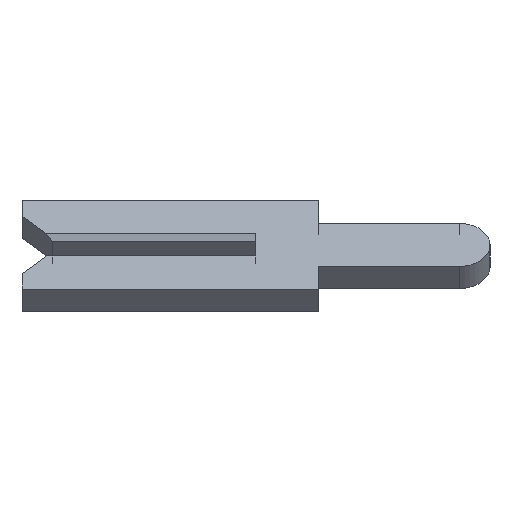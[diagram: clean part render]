
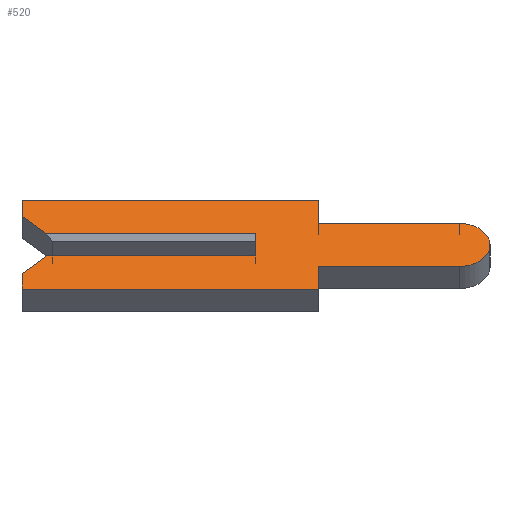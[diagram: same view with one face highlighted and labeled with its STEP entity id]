
A CAD part, left-side view. The second image highlights one B-rep face of the part: STEP entity #520.
In plain terms, the highlighted face is planar.
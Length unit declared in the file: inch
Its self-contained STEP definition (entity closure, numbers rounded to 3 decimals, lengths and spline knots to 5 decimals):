
#5 = VERTEX_POINT ( 'NONE', #179 ) ;
#6 = EDGE_CURVE ( 'NONE', #775, #765, #870, .T. ) ;
#57 = LINE ( 'NONE', #976, #354 ) ;
#66 = DIRECTION ( 'NONE',  ( 0., 0., 1. ) ) ;
#78 = ORIENTED_EDGE ( 'NONE', *, *, #1121, .F. ) ;
#79 = VECTOR ( 'NONE', #904, 39.37008 ) ;
#104 = LINE ( 'NONE', #142, #143 ) ;
#142 = CARTESIAN_POINT ( 'NONE',  ( -0.01, -0.1305, -0.01 ) ) ;
#143 = VECTOR ( 'NONE', #696, 39.37008 ) ;
#173 = VERTEX_POINT ( 'NONE', #862 ) ;
#179 = CARTESIAN_POINT ( 'NONE',  ( -0.01, -0.04, 0.0195 ) ) ;
#180 = EDGE_CURVE ( 'NONE', #813, #1095, #745, .T. ) ;
#182 = CARTESIAN_POINT ( 'NONE',  ( -0.01, 0.15, 0.026 ) ) ;
#183 = CARTESIAN_POINT ( 'NONE',  ( -0.01, 0., -0.01 ) ) ;
#207 = PLANE ( 'NONE',  #774 ) ;
#228 = ORIENTED_EDGE ( 'NONE', *, *, #690, .F. ) ;
#273 = ORIENTED_EDGE ( 'NONE', *, *, #647, .F. ) ;
#275 = VECTOR ( 'NONE', #646, 39.37008 ) ;
#296 = VERTEX_POINT ( 'NONE', #309 ) ;
#297 = DIRECTION ( 'NONE',  ( 0., 1., 0. ) ) ;
#301 = AXIS2_PLACEMENT_3D ( 'NONE', #403, #713, #1170 ) ;
#309 = CARTESIAN_POINT ( 'NONE',  ( -0.01, 0.134, -0.01 ) ) ;
#322 = LINE ( 'NONE', #568, #867 ) ;
#323 = VERTEX_POINT ( 'NONE', #183 ) ;
#328 = DIRECTION ( 'NONE',  ( 0., 0., -1. ) ) ;
#346 = DIRECTION ( 'NONE',  ( 0., 0., 1. ) ) ;
#347 = VECTOR ( 'NONE', #406, 39.37008 ) ;
#348 = EDGE_CURVE ( 'NONE', #813, #601, #396, .T. ) ;
#350 = CARTESIAN_POINT ( 'NONE',  ( -0.01, -0.04, -0.04 ) ) ;
#354 = VECTOR ( 'NONE', #297, 39.37008 ) ;
#396 = LINE ( 'NONE', #1088, #1041 ) ;
#403 = CARTESIAN_POINT ( 'NONE',  ( -0.01, -0.1305, 0. ) ) ;
#406 = DIRECTION ( 'NONE',  ( 0., 0.707, 0.707 ) ) ;
#424 = LINE ( 'NONE', #571, #457 ) ;
#455 = CARTESIAN_POINT ( 'NONE',  ( -0.01, -0.04, 0.04 ) ) ;
#457 = VECTOR ( 'NONE', #1120, 39.37008 ) ;
#462 = ORIENTED_EDGE ( 'NONE', *, *, #1383, .F. ) ;
#465 = CARTESIAN_POINT ( 'NONE',  ( -0.01, 0.15, -0.026 ) ) ;
#471 = VECTOR ( 'NONE', #803, 39.37008 ) ;
#473 = EDGE_CURVE ( 'NONE', #849, #1126, #57, .T. ) ;
#490 = CARTESIAN_POINT ( 'NONE',  ( -0.01, 0.1305, 0.0065 ) ) ;
#500 = DIRECTION ( 'NONE',  ( 0., 0., 1. ) ) ;
#520 = ADVANCED_FACE ( 'NONE', ( #1239 ), #207, .F. ) ;
#532 = EDGE_LOOP ( 'NONE', ( #1036, #462, #78, #1132, #228, #1076, #273, #1227, #930, #1108, #1195, #794, #534, #1018 ) ) ;
#534 = ORIENTED_EDGE ( 'NONE', *, *, #1335, .F. ) ;
#551 = EDGE_CURVE ( 'NONE', #670, #296, #1303, .T. ) ;
#566 = EDGE_CURVE ( 'NONE', #173, #1384, #1125, .T. ) ;
#568 = CARTESIAN_POINT ( 'NONE',  ( -0.01, 0.15, -0.026 ) ) ;
#571 = CARTESIAN_POINT ( 'NONE',  ( -0.01, -0.04, 0.04 ) ) ;
#585 = VECTOR ( 'NONE', #66, 39.37008 ) ;
#601 = VERTEX_POINT ( 'NONE', #767 ) ;
#646 = DIRECTION ( 'NONE',  ( 0., 1., 0. ) ) ;
#647 = EDGE_CURVE ( 'NONE', #1384, #849, #1158, .T. ) ;
#670 = VERTEX_POINT ( 'NONE', #465 ) ;
#682 = CARTESIAN_POINT ( 'NONE',  ( -0.01, -0.1305, 0.0195 ) ) ;
#690 = EDGE_CURVE ( 'NONE', #1126, #670, #322, .T. ) ;
#696 = DIRECTION ( 'NONE',  ( 0., -1., 0. ) ) ;
#713 = DIRECTION ( 'NONE',  ( 1., 0., 0. ) ) ;
#714 = VECTOR ( 'NONE', #1310, 39.37008 ) ;
#719 = VERTEX_POINT ( 'NONE', #682 ) ;
#730 = LINE ( 'NONE', #182, #822 ) ;
#745 = LINE ( 'NONE', #490, #347 ) ;
#764 = CARTESIAN_POINT ( 'NONE',  ( -0.01, -0.1305, 0. ) ) ;
#765 = VERTEX_POINT ( 'NONE', #455 ) ;
#767 = CARTESIAN_POINT ( 'NONE',  ( -0.01, 0., 0.01 ) ) ;
#768 = CIRCLE ( 'NONE', #301, 0.0195 ) ;
#771 = DIRECTION ( 'NONE',  ( 1., 0., 0. ) ) ;
#774 = AXIS2_PLACEMENT_3D ( 'NONE', #764, #771, #328 ) ;
#775 = VERTEX_POINT ( 'NONE', #1336 ) ;
#794 = ORIENTED_EDGE ( 'NONE', *, *, #6, .F. ) ;
#803 = DIRECTION ( 'NONE',  ( 0., -1., 0. ) ) ;
#813 = VERTEX_POINT ( 'NONE', #1130 ) ;
#822 = VECTOR ( 'NONE', #500, 39.37008 ) ;
#825 = EDGE_CURVE ( 'NONE', #5, #719, #932, .T. ) ;
#849 = VERTEX_POINT ( 'NONE', #350 ) ;
#862 = CARTESIAN_POINT ( 'NONE',  ( -0.01, -0.1305, -0.0195 ) ) ;
#867 = VECTOR ( 'NONE', #346, 39.37008 ) ;
#870 = LINE ( 'NONE', #1063, #936 ) ;
#874 = CARTESIAN_POINT ( 'NONE',  ( -0.01, 0.1305, -0.0065 ) ) ;
#895 = EDGE_CURVE ( 'NONE', #765, #5, #424, .T. ) ;
#904 = DIRECTION ( 'NONE',  ( 0., 0., -1. ) ) ;
#909 = CARTESIAN_POINT ( 'NONE',  ( -0.01, -0.04, -0.04 ) ) ;
#930 = ORIENTED_EDGE ( 'NONE', *, *, #1309, .F. ) ;
#932 = LINE ( 'NONE', #1347, #471 ) ;
#936 = VECTOR ( 'NONE', #1171, 39.37008 ) ;
#937 = CARTESIAN_POINT ( 'NONE',  ( -0.01, 0.15, -0.04 ) ) ;
#976 = CARTESIAN_POINT ( 'NONE',  ( -0.01, 0.15, -0.04 ) ) ;
#996 = LINE ( 'NONE', #1181, #585 ) ;
#1018 = ORIENTED_EDGE ( 'NONE', *, *, #180, .F. ) ;
#1036 = ORIENTED_EDGE ( 'NONE', *, *, #348, .T. ) ;
#1041 = VECTOR ( 'NONE', #1187, 39.37008 ) ;
#1063 = CARTESIAN_POINT ( 'NONE',  ( -0.01, 0.15, 0.04 ) ) ;
#1076 = ORIENTED_EDGE ( 'NONE', *, *, #473, .F. ) ;
#1088 = CARTESIAN_POINT ( 'NONE',  ( -0.01, 0.15, 0.01 ) ) ;
#1095 = VERTEX_POINT ( 'NONE', #1361 ) ;
#1102 = CARTESIAN_POINT ( 'NONE',  ( -0.01, -0.04, -0.0195 ) ) ;
#1108 = ORIENTED_EDGE ( 'NONE', *, *, #825, .F. ) ;
#1120 = DIRECTION ( 'NONE',  ( 0., 0., -1. ) ) ;
#1121 = EDGE_CURVE ( 'NONE', #296, #323, #104, .T. ) ;
#1125 = LINE ( 'NONE', #1102, #275 ) ;
#1126 = VERTEX_POINT ( 'NONE', #937 ) ;
#1130 = CARTESIAN_POINT ( 'NONE',  ( -0.01, 0.134, 0.01 ) ) ;
#1132 = ORIENTED_EDGE ( 'NONE', *, *, #551, .F. ) ;
#1158 = LINE ( 'NONE', #909, #79 ) ;
#1170 = DIRECTION ( 'NONE',  ( 0., 0., -1. ) ) ;
#1171 = DIRECTION ( 'NONE',  ( 0., -1., 0. ) ) ;
#1181 = CARTESIAN_POINT ( 'NONE',  ( -0.01, 0., 0.0065 ) ) ;
#1187 = DIRECTION ( 'NONE',  ( 0., -1., 0. ) ) ;
#1195 = ORIENTED_EDGE ( 'NONE', *, *, #895, .F. ) ;
#1227 = ORIENTED_EDGE ( 'NONE', *, *, #566, .F. ) ;
#1239 = FACE_OUTER_BOUND ( 'NONE', #532, .T. ) ;
#1303 = LINE ( 'NONE', #874, #714 ) ;
#1309 = EDGE_CURVE ( 'NONE', #719, #173, #768, .T. ) ;
#1310 = DIRECTION ( 'NONE',  ( 0., -0.707, 0.707 ) ) ;
#1335 = EDGE_CURVE ( 'NONE', #1095, #775, #730, .T. ) ;
#1336 = CARTESIAN_POINT ( 'NONE',  ( -0.01, 0.15, 0.04 ) ) ;
#1347 = CARTESIAN_POINT ( 'NONE',  ( -0.01, -0.04, 0.0195 ) ) ;
#1361 = CARTESIAN_POINT ( 'NONE',  ( -0.01, 0.15, 0.026 ) ) ;
#1383 = EDGE_CURVE ( 'NONE', #323, #601, #996, .T. ) ;
#1384 = VERTEX_POINT ( 'NONE', #1385 ) ;
#1385 = CARTESIAN_POINT ( 'NONE',  ( -0.01, -0.04, -0.0195 ) ) ;
